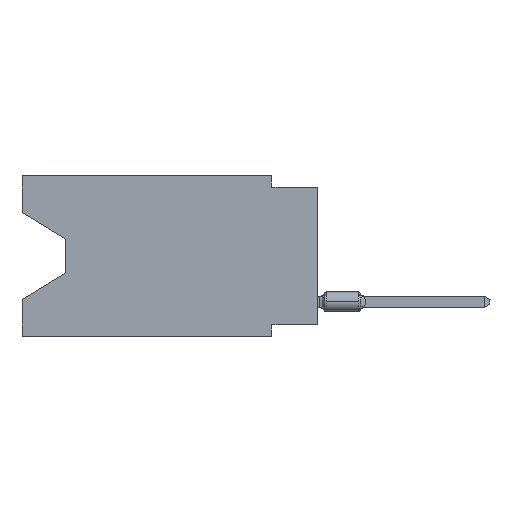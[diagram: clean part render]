
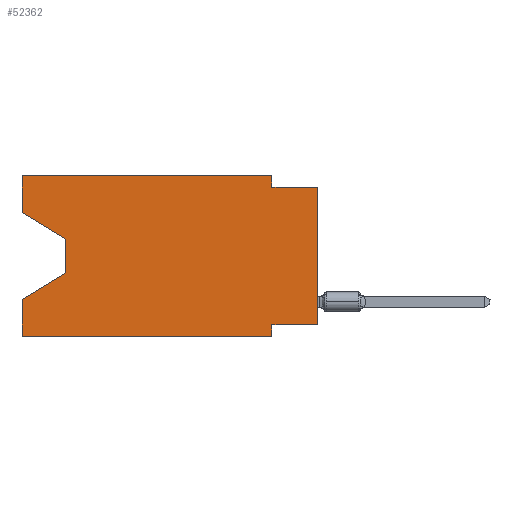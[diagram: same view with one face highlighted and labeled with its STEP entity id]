
A CAD part, left-side view. The second image highlights one B-rep face of the part: STEP entity #52362.
In plain terms, the highlighted planar face has unit normal (-1, 0, 0).
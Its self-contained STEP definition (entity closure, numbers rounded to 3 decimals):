
#3374 = DIRECTION ( 'NONE',  ( 0., -0.855, -0.519 ) ) ;
#5505 = CARTESIAN_POINT ( 'NONE',  ( 0., 16.383, 0. ) ) ;
#6287 = DIRECTION ( 'NONE',  ( 0., -1., 0. ) ) ;
#6535 = VECTOR ( 'NONE', #63453, 1000. ) ;
#11728 = CARTESIAN_POINT ( 'NONE',  ( 0., 16.383, 0. ) ) ;
#12242 = LINE ( 'NONE', #11728, #34571 ) ;
#15381 = VERTEX_POINT ( 'NONE', #76099 ) ;
#15470 = CARTESIAN_POINT ( 'NONE',  ( 0., 2.54, -8.255 ) ) ;
#15906 = CARTESIAN_POINT ( 'NONE',  ( 0., 0., -0.635 ) ) ;
#17707 = EDGE_CURVE ( 'NONE', #68126, #30519, #12242, .T. ) ;
#18692 = DIRECTION ( 'NONE',  ( 0., 0., 1. ) ) ;
#20731 = CARTESIAN_POINT ( 'NONE',  ( 0., 16.383, -6.852 ) ) ;
#20932 = VERTEX_POINT ( 'NONE', #27182 ) ;
#23144 = ORIENTED_EDGE ( 'NONE', *, *, #89154, .F. ) ;
#23523 = VECTOR ( 'NONE', #18692, 1000. ) ;
#24170 = VECTOR ( 'NONE', #80101, 1000. ) ;
#24305 = FACE_OUTER_BOUND ( 'NONE', #98475, .T. ) ;
#24468 = VECTOR ( 'NONE', #87701, 1000. ) ;
#26288 = EDGE_CURVE ( 'NONE', #91675, #49535, #38017, .T. ) ;
#27182 = CARTESIAN_POINT ( 'NONE',  ( 0., 2.54, 0. ) ) ;
#28682 = VECTOR ( 'NONE', #6287, 1000. ) ;
#30519 = VERTEX_POINT ( 'NONE', #20731 ) ;
#30653 = VECTOR ( 'NONE', #43850, 1000. ) ;
#31136 = CARTESIAN_POINT ( 'NONE',  ( 0., 2.54, -8.89 ) ) ;
#32991 = EDGE_CURVE ( 'NONE', #15381, #30519, #61789, .T. ) ;
#33710 = DIRECTION ( 'NONE',  ( 0., 0., -1. ) ) ;
#34571 = VECTOR ( 'NONE', #91205, 1000. ) ;
#35726 = EDGE_CURVE ( 'NONE', #49535, #56118, #39934, .T. ) ;
#35816 = VERTEX_POINT ( 'NONE', #73670 ) ;
#38017 = LINE ( 'NONE', #79509, #46439 ) ;
#38423 = DIRECTION ( 'NONE',  ( 0., 0.855, -0.519 ) ) ;
#39035 = DIRECTION ( 'NONE',  ( 0., 1., 0. ) ) ;
#39934 = LINE ( 'NONE', #31136, #24468 ) ;
#41342 = EDGE_CURVE ( 'NONE', #72211, #84423, #64939, .T. ) ;
#43369 = CARTESIAN_POINT ( 'NONE',  ( 0., 16.383, -2.038 ) ) ;
#43850 = DIRECTION ( 'NONE',  ( 0., 0., 1. ) ) ;
#45407 = CARTESIAN_POINT ( 'NONE',  ( 0., 0., 0. ) ) ;
#45624 = ORIENTED_EDGE ( 'NONE', *, *, #78011, .T. ) ;
#46439 = VECTOR ( 'NONE', #39035, 1000. ) ;
#46494 = CARTESIAN_POINT ( 'NONE',  ( 0., 16.383, -8.89 ) ) ;
#47385 = CARTESIAN_POINT ( 'NONE',  ( 0., 0., -0.635 ) ) ;
#47453 = CARTESIAN_POINT ( 'NONE',  ( 0., 16.383, -8.89 ) ) ;
#48433 = VERTEX_POINT ( 'NONE', #15906 ) ;
#49364 = CARTESIAN_POINT ( 'NONE',  ( 0., 16.383, 0. ) ) ;
#49535 = VERTEX_POINT ( 'NONE', #15470 ) ;
#50935 = ORIENTED_EDGE ( 'NONE', *, *, #26288, .F. ) ;
#51036 = CARTESIAN_POINT ( 'NONE',  ( 0., 13.97, -3.505 ) ) ;
#51982 = AXIS2_PLACEMENT_3D ( 'NONE', #61753, #93431, #77843 ) ;
#52362 = ADVANCED_FACE ( 'NONE', ( #24305 ), #69549, .F. ) ;
#52637 = CARTESIAN_POINT ( 'NONE',  ( 0., 0., -8.255 ) ) ;
#53756 = LINE ( 'NONE', #46494, #59722 ) ;
#55176 = LINE ( 'NONE', #47385, #6535 ) ;
#56118 = VERTEX_POINT ( 'NONE', #61302 ) ;
#56496 = ORIENTED_EDGE ( 'NONE', *, *, #17707, .F. ) ;
#57259 = LINE ( 'NONE', #88940, #24170 ) ;
#59722 = VECTOR ( 'NONE', #100500, 1000. ) ;
#61302 = CARTESIAN_POINT ( 'NONE',  ( 0., 2.54, -8.89 ) ) ;
#61753 = CARTESIAN_POINT ( 'NONE',  ( 0., 16.383, 0. ) ) ;
#61789 = LINE ( 'NONE', #62803, #67344 ) ;
#62363 = CARTESIAN_POINT ( 'NONE',  ( 0., 16.383, -2.038 ) ) ;
#62803 = CARTESIAN_POINT ( 'NONE',  ( 0., 13.97, -5.385 ) ) ;
#63453 = DIRECTION ( 'NONE',  ( 0., -1., 0. ) ) ;
#64244 = ORIENTED_EDGE ( 'NONE', *, *, #41342, .F. ) ;
#64939 = LINE ( 'NONE', #49364, #23523 ) ;
#67344 = VECTOR ( 'NONE', #38423, 1000. ) ;
#68126 = VERTEX_POINT ( 'NONE', #47453 ) ;
#69549 = PLANE ( 'NONE',  #51982 ) ;
#70675 = CARTESIAN_POINT ( 'NONE',  ( 0., 16.383, 0. ) ) ;
#71113 = ORIENTED_EDGE ( 'NONE', *, *, #94784, .T. ) ;
#71636 = ORIENTED_EDGE ( 'NONE', *, *, #79009, .T. ) ;
#72211 = VERTEX_POINT ( 'NONE', #62363 ) ;
#72992 = EDGE_CURVE ( 'NONE', #91675, #48433, #84870, .T. ) ;
#73483 = ORIENTED_EDGE ( 'NONE', *, *, #32991, .T. ) ;
#73670 = CARTESIAN_POINT ( 'NONE',  ( 0., 2.54, -0.635 ) ) ;
#74519 = LINE ( 'NONE', #43369, #86131 ) ;
#74723 = LINE ( 'NONE', #89811, #87856 ) ;
#76099 = CARTESIAN_POINT ( 'NONE',  ( 0., 13.97, -5.385 ) ) ;
#76390 = ORIENTED_EDGE ( 'NONE', *, *, #86502, .F. ) ;
#77411 = ORIENTED_EDGE ( 'NONE', *, *, #72992, .T. ) ;
#77843 = DIRECTION ( 'NONE',  ( 0., 0., -1. ) ) ;
#78011 = EDGE_CURVE ( 'NONE', #72211, #101420, #74519, .T. ) ;
#79009 = EDGE_CURVE ( 'NONE', #68126, #56118, #53756, .T. ) ;
#79509 = CARTESIAN_POINT ( 'NONE',  ( 0., 0., -8.255 ) ) ;
#80101 = DIRECTION ( 'NONE',  ( 0., 0., -1. ) ) ;
#84423 = VERTEX_POINT ( 'NONE', #5505 ) ;
#84870 = LINE ( 'NONE', #45407, #30653 ) ;
#86131 = VECTOR ( 'NONE', #3374, 1000. ) ;
#86502 = EDGE_CURVE ( 'NONE', #84423, #20932, #100800, .T. ) ;
#87701 = DIRECTION ( 'NONE',  ( 0., 0., -1. ) ) ;
#87856 = VECTOR ( 'NONE', #33710, 1000. ) ;
#88457 = ORIENTED_EDGE ( 'NONE', *, *, #92970, .F. ) ;
#88940 = CARTESIAN_POINT ( 'NONE',  ( 0., 2.54, 0. ) ) ;
#89154 = EDGE_CURVE ( 'NONE', #20932, #35816, #57259, .T. ) ;
#89811 = CARTESIAN_POINT ( 'NONE',  ( 0., 13.97, -3.505 ) ) ;
#91205 = DIRECTION ( 'NONE',  ( 0., 0., 1. ) ) ;
#91675 = VERTEX_POINT ( 'NONE', #52637 ) ;
#92970 = EDGE_CURVE ( 'NONE', #35816, #48433, #55176, .T. ) ;
#93431 = DIRECTION ( 'NONE',  ( 1., 0., 0. ) ) ;
#94784 = EDGE_CURVE ( 'NONE', #101420, #15381, #74723, .T. ) ;
#98475 = EDGE_LOOP ( 'NONE', ( #45624, #71113, #73483, #56496, #71636, #101620, #50935, #77411, #88457, #23144, #76390, #64244 ) ) ;
#100500 = DIRECTION ( 'NONE',  ( 0., -1., 0. ) ) ;
#100800 = LINE ( 'NONE', #70675, #28682 ) ;
#101420 = VERTEX_POINT ( 'NONE', #51036 ) ;
#101620 = ORIENTED_EDGE ( 'NONE', *, *, #35726, .F. ) ;
